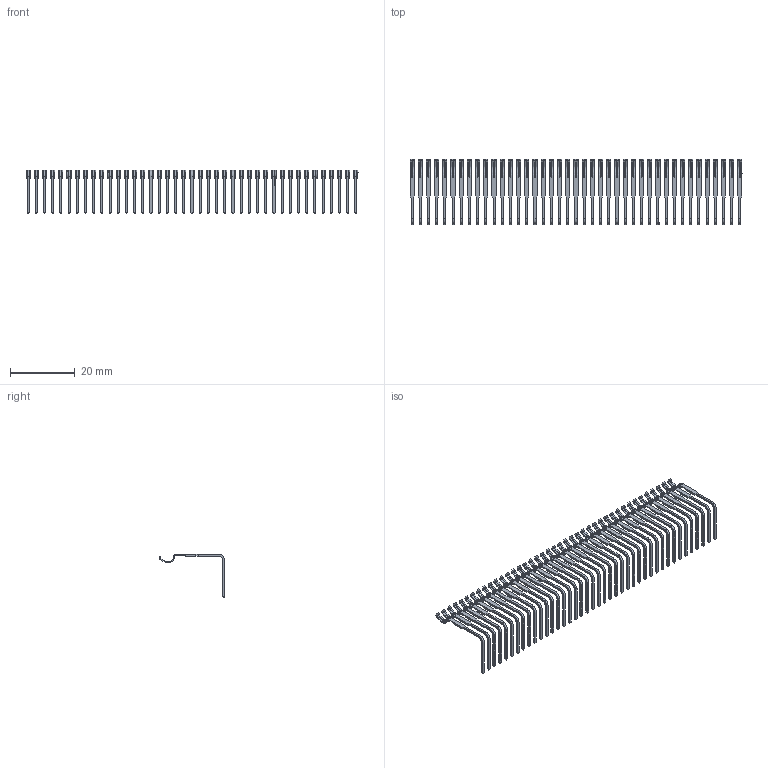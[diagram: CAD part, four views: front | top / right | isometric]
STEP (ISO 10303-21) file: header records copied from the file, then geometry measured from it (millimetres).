
FILE_DESCRIPTION (( 'STEP AP203' ), '1' );
FILE_NAME ('345-041-558-412.STEP', '2019-10-10T16:18:25', ( '' ), ( '' ), 'SwSTEP 2.0', 'SolidWorks 2016', '' );
FILE_SCHEMA (( 'CONFIG_CONTROL_DESIGN' ));
Length unit declared in the file: inch
Products named in the file (3): 345 Part_0.110 Offset - Side Mount; 345-292-001_558 Tail - 2; 345-041-558-412
Assembly tree (42 placements, depth 2):
  345-041-558-412
    345 Part_0.110 Offset - Side Mount
    345-292-001_558 Tail - 2  x41
Bounding box: 102.87 x 20.26 x 13.53 mm (x, y, z)
Volume: 606.1 mm3; surface area: 4101.3 mm2
Topology: 41 solids, 41 shells, 1804 faces, 5248 edges, 3444 vertices
Faces by surface type: plane 1148, cylinder 656
Entity records: 31211 total; most frequent: CARTESIAN_POINT 5415, ORIENTED_EDGE 5390, DIRECTION 4729, EDGE_CURVE 2695, LINE 2399, VECTOR 2399, VERTEX_POINT 1794, AXIS2_PLACEMENT_3D 1165
